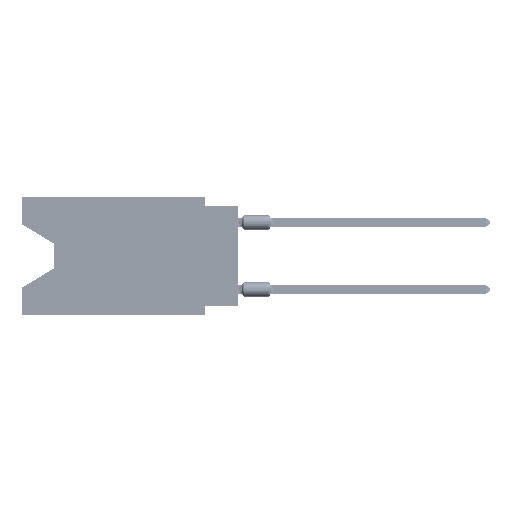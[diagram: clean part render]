
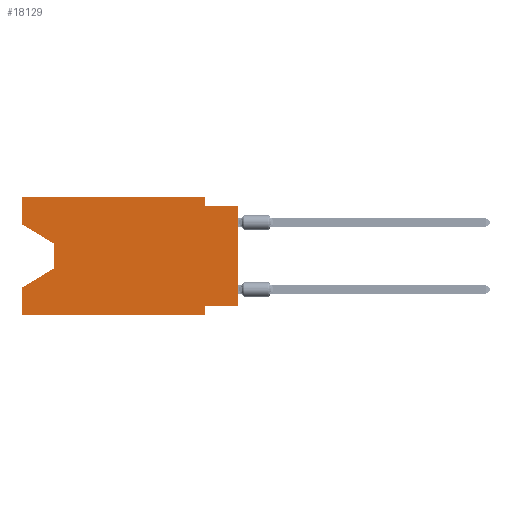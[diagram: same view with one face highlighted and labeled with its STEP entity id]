
A CAD part, left-side view. The second image highlights one B-rep face of the part: STEP entity #18129.
In plain terms, the highlighted planar face has unit normal (-1, 0, 0).
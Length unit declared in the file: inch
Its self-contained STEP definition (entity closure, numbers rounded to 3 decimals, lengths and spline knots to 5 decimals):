
#456 = EDGE_CURVE ( 'NONE', #13824, #80190, #50121, .T. ) ;
#2419 = DIRECTION ( 'NONE',  ( 0., -1., 0. ) ) ;
#2720 = EDGE_CURVE ( 'NONE', #89560, #38213, #15955, .T. ) ;
#3138 = EDGE_CURVE ( 'NONE', #76605, #6597, #15843, .T. ) ;
#3324 = CARTESIAN_POINT ( 'NONE',  ( 0., 0.1, -0.35 ) ) ;
#3922 = VECTOR ( 'NONE', #15364, 39.37008 ) ;
#4354 = ORIENTED_EDGE ( 'NONE', *, *, #70201, .T. ) ;
#6046 = ORIENTED_EDGE ( 'NONE', *, *, #21653, .T. ) ;
#6463 = VECTOR ( 'NONE', #56114, 39.37008 ) ;
#6597 = VERTEX_POINT ( 'NONE', #49749 ) ;
#7350 = CARTESIAN_POINT ( 'NONE',  ( 0., 0.645, 0. ) ) ;
#7650 = VERTEX_POINT ( 'NONE', #20436 ) ;
#8418 = LINE ( 'NONE', #78718, #60600 ) ;
#8923 = DIRECTION ( 'NONE',  ( 0., 0., 1. ) ) ;
#9580 = LINE ( 'NONE', #23834, #69168 ) ;
#10867 = CARTESIAN_POINT ( 'NONE',  ( 0., 0.1, -0.025 ) ) ;
#10912 = CARTESIAN_POINT ( 'NONE',  ( 0., 0.55, -0.212 ) ) ;
#12716 = VERTEX_POINT ( 'NONE', #84495 ) ;
#12892 = CARTESIAN_POINT ( 'NONE',  ( 0., 0.645, 0. ) ) ;
#13824 = VERTEX_POINT ( 'NONE', #53276 ) ;
#14136 = LINE ( 'NONE', #35257, #21682 ) ;
#15023 = DIRECTION ( 'NONE',  ( 0., -0.855, -0.519 ) ) ;
#15364 = DIRECTION ( 'NONE',  ( 0., 0., 1. ) ) ;
#15843 = LINE ( 'NONE', #71870, #48701 ) ;
#15955 = LINE ( 'NONE', #30198, #35412 ) ;
#18129 = ADVANCED_FACE ( 'NONE', ( #84095 ), #49179, .F. ) ;
#18796 = VERTEX_POINT ( 'NONE', #47134 ) ;
#20160 = VERTEX_POINT ( 'NONE', #36883 ) ;
#20436 = CARTESIAN_POINT ( 'NONE',  ( 0., 0.645, -0.08025 ) ) ;
#21653 = EDGE_CURVE ( 'NONE', #12716, #80602, #8418, .T. ) ;
#21682 = VECTOR ( 'NONE', #15023, 39.37008 ) ;
#22474 = VERTEX_POINT ( 'NONE', #44377 ) ;
#23834 = CARTESIAN_POINT ( 'NONE',  ( 0., 0., -0.325 ) ) ;
#25053 = ORIENTED_EDGE ( 'NONE', *, *, #33796, .F. ) ;
#25636 = AXIS2_PLACEMENT_3D ( 'NONE', #7350, #42296, #70305 ) ;
#27365 = EDGE_CURVE ( 'NONE', #20160, #18796, #48013, .T. ) ;
#29263 = ORIENTED_EDGE ( 'NONE', *, *, #62945, .F. ) ;
#30014 = ORIENTED_EDGE ( 'NONE', *, *, #90339, .F. ) ;
#30198 = CARTESIAN_POINT ( 'NONE',  ( 0., 0.1, 0. ) ) ;
#30651 = ORIENTED_EDGE ( 'NONE', *, *, #44673, .F. ) ;
#30900 = LINE ( 'NONE', #65374, #45466 ) ;
#33796 = EDGE_CURVE ( 'NONE', #38213, #6597, #80111, .T. ) ;
#35257 = CARTESIAN_POINT ( 'NONE',  ( 0., 0.645, -0.08025 ) ) ;
#35412 = VECTOR ( 'NONE', #36630, 39.37008 ) ;
#36630 = DIRECTION ( 'NONE',  ( 0., 0., -1. ) ) ;
#36883 = CARTESIAN_POINT ( 'NONE',  ( 0., 0.645, -0.35 ) ) ;
#37547 = LINE ( 'NONE', #87622, #44703 ) ;
#38213 = VERTEX_POINT ( 'NONE', #10867 ) ;
#41128 = VECTOR ( 'NONE', #74544, 39.37008 ) ;
#42296 = DIRECTION ( 'NONE',  ( 1., 0., 0. ) ) ;
#43587 = DIRECTION ( 'NONE',  ( 0., 1., 0. ) ) ;
#44377 = CARTESIAN_POINT ( 'NONE',  ( 0., 0.645, 0. ) ) ;
#44673 = EDGE_CURVE ( 'NONE', #22474, #89560, #30900, .T. ) ;
#44703 = VECTOR ( 'NONE', #71972, 39.37008 ) ;
#45466 = VECTOR ( 'NONE', #2419, 39.37008 ) ;
#46512 = CARTESIAN_POINT ( 'NONE',  ( 0., 0., -0.025 ) ) ;
#47134 = CARTESIAN_POINT ( 'NONE',  ( 0., 0.645, -0.26975 ) ) ;
#47610 = ORIENTED_EDGE ( 'NONE', *, *, #3138, .T. ) ;
#48013 = LINE ( 'NONE', #76041, #3922 ) ;
#48701 = VECTOR ( 'NONE', #8923, 39.37008 ) ;
#49179 = PLANE ( 'NONE',  #25636 ) ;
#49322 = DIRECTION ( 'NONE',  ( 0., 0., -1. ) ) ;
#49749 = CARTESIAN_POINT ( 'NONE',  ( 0., 0., -0.025 ) ) ;
#50121 = LINE ( 'NONE', #83283, #6463 ) ;
#50142 = EDGE_CURVE ( 'NONE', #80602, #18796, #68841, .T. ) ;
#53236 = VECTOR ( 'NONE', #89547, 39.37008 ) ;
#53276 = CARTESIAN_POINT ( 'NONE',  ( 0., 0.1, -0.325 ) ) ;
#56114 = DIRECTION ( 'NONE',  ( 0., 0., -1. ) ) ;
#56811 = ORIENTED_EDGE ( 'NONE', *, *, #27365, .F. ) ;
#57675 = ORIENTED_EDGE ( 'NONE', *, *, #456, .F. ) ;
#60600 = VECTOR ( 'NONE', #49322, 39.37008 ) ;
#62945 = EDGE_CURVE ( 'NONE', #7650, #22474, #69357, .T. ) ;
#65374 = CARTESIAN_POINT ( 'NONE',  ( 0., 0.645, 0. ) ) ;
#68841 = LINE ( 'NONE', #89988, #53236 ) ;
#69168 = VECTOR ( 'NONE', #43587, 39.37008 ) ;
#69357 = LINE ( 'NONE', #12892, #83665 ) ;
#70201 = EDGE_CURVE ( 'NONE', #20160, #80190, #37547, .T. ) ;
#70305 = DIRECTION ( 'NONE',  ( 0., 0., -1. ) ) ;
#71870 = CARTESIAN_POINT ( 'NONE',  ( 0., 0., 0. ) ) ;
#71972 = DIRECTION ( 'NONE',  ( 0., -1., 0. ) ) ;
#72751 = EDGE_LOOP ( 'NONE', ( #76508, #6046, #78742, #56811, #4354, #57675, #30014, #47610, #25053, #89120, #30651, #29263 ) ) ;
#73565 = EDGE_CURVE ( 'NONE', #7650, #12716, #14136, .T. ) ;
#74544 = DIRECTION ( 'NONE',  ( 0., -1., 0. ) ) ;
#75784 = CARTESIAN_POINT ( 'NONE',  ( 0., 0., -0.325 ) ) ;
#76041 = CARTESIAN_POINT ( 'NONE',  ( 0., 0.645, 0. ) ) ;
#76508 = ORIENTED_EDGE ( 'NONE', *, *, #73565, .T. ) ;
#76605 = VERTEX_POINT ( 'NONE', #75784 ) ;
#78713 = CARTESIAN_POINT ( 'NONE',  ( 0., 0.1, 0. ) ) ;
#78718 = CARTESIAN_POINT ( 'NONE',  ( 0., 0.55, -0.138 ) ) ;
#78742 = ORIENTED_EDGE ( 'NONE', *, *, #50142, .T. ) ;
#80111 = LINE ( 'NONE', #46512, #41128 ) ;
#80190 = VERTEX_POINT ( 'NONE', #3324 ) ;
#80602 = VERTEX_POINT ( 'NONE', #10912 ) ;
#83196 = DIRECTION ( 'NONE',  ( 0., 0., 1. ) ) ;
#83283 = CARTESIAN_POINT ( 'NONE',  ( 0., 0.1, -0.35 ) ) ;
#83665 = VECTOR ( 'NONE', #83196, 39.37008 ) ;
#84095 = FACE_OUTER_BOUND ( 'NONE', #72751, .T. ) ;
#84495 = CARTESIAN_POINT ( 'NONE',  ( 0., 0.55, -0.138 ) ) ;
#87622 = CARTESIAN_POINT ( 'NONE',  ( 0., 0.645, -0.35 ) ) ;
#89120 = ORIENTED_EDGE ( 'NONE', *, *, #2720, .F. ) ;
#89547 = DIRECTION ( 'NONE',  ( 0., 0.855, -0.519 ) ) ;
#89560 = VERTEX_POINT ( 'NONE', #78713 ) ;
#89988 = CARTESIAN_POINT ( 'NONE',  ( 0., 0.55, -0.212 ) ) ;
#90339 = EDGE_CURVE ( 'NONE', #76605, #13824, #9580, .T. ) ;
